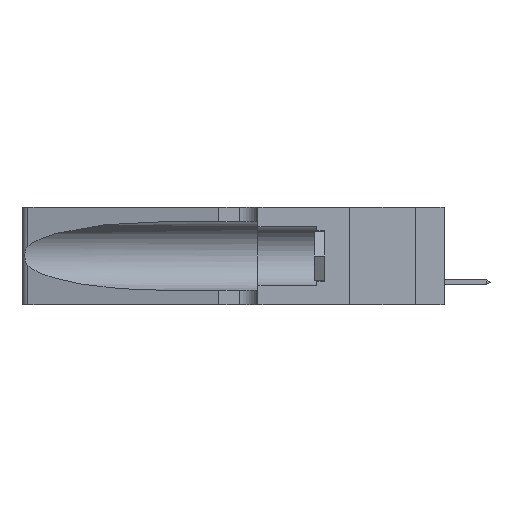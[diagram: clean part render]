
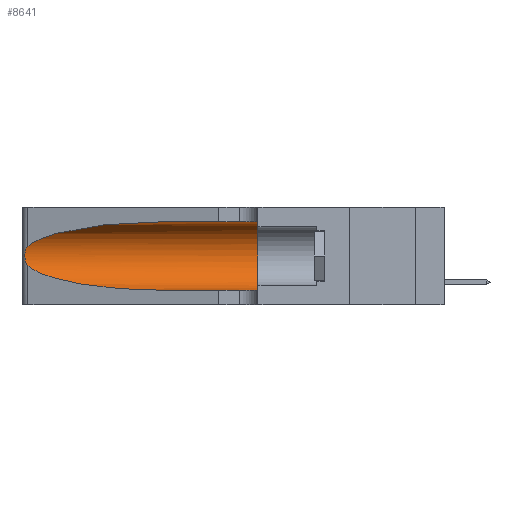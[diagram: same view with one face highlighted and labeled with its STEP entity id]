
A CAD part, left-side view. The second image highlights one B-rep face of the part: STEP entity #8641.
In plain terms, the highlighted cylindrical face has radius 3.308 mm (diameter 6.617 mm), a partial arc.
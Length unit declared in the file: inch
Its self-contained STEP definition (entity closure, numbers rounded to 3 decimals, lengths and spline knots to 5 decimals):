
#353 =( BOUNDED_CURVE ( )  B_SPLINE_CURVE ( 3, ( #4909, #16936, #8805, #553 ),
 .UNSPECIFIED., .F., .T. ) 
 B_SPLINE_CURVE_WITH_KNOTS ( ( 4, 4 ),
 ( 3.44316, 4.71239 ),
 .UNSPECIFIED. ) 
 CURVE ( )  GEOMETRIC_REPRESENTATION_ITEM ( )  RATIONAL_B_SPLINE_CURVE ( ( 1., 0.87, 0.87, 1. ) ) 
 REPRESENTATION_ITEM ( '' )  );
#553 = CARTESIAN_POINT ( 'NONE',  ( 0.1305, 0.72297, 0.05475 ) ) ;
#619 = ORIENTED_EDGE ( 'NONE', *, *, #15987, .F. ) ;
#901 = DIRECTION ( 'NONE',  ( 0., 0., -1. ) ) ;
#963 = CARTESIAN_POINT ( 'NONE',  ( 0.25789, 1.23486, 0.15765 ) ) ;
#1124 = CARTESIAN_POINT ( 'NONE',  ( 0.18966, 0.96281, 0.31525 ) ) ;
#1194 = ORIENTED_EDGE ( 'NONE', *, *, #21502, .F. ) ;
#1663 = VERTEX_POINT ( 'NONE', #10010 ) ;
#2228 = CARTESIAN_POINT ( 'NONE',  ( 0.1305, 0.35, 0.05475 ) ) ;
#2381 = DIRECTION ( 'NONE',  ( 0., -1., 0. ) ) ;
#2881 = CARTESIAN_POINT ( 'NONE',  ( 0.1305, 1.61858, 0.185 ) ) ;
#3036 = CARTESIAN_POINT ( 'NONE',  ( 0.25487, 1.22718, 0.22369 ) ) ;
#3123 = CARTESIAN_POINT ( 'NONE',  ( 0.26075, 1.23896, 0.19203 ) ) ;
#3367 = CARTESIAN_POINT ( 'NONE',  ( 0.25487, 1.22718, 0.22369 ) ) ;
#3397 = CARTESIAN_POINT ( 'NONE',  ( 0.26075, 1.23896, 0.178 ) ) ;
#3483 = LINE ( 'NONE', #20810, #13830 ) ;
#3526 = EDGE_LOOP ( 'NONE', ( #8559, #12706, #19933, #14990, #1194, #619 ) ) ;
#3646 = FACE_OUTER_BOUND ( 'NONE', #3526, .T. ) ;
#4675 =( BOUNDED_CURVE ( )  B_SPLINE_CURVE ( 3, ( #25642, #1124, #13586, #3367 ),
 .UNSPECIFIED., .F., .F. ) 
 B_SPLINE_CURVE_WITH_KNOTS ( ( 4, 4 ),
 ( 1.5708, 2.84003 ),
 .UNSPECIFIED. ) 
 CURVE ( )  GEOMETRIC_REPRESENTATION_ITEM ( )  RATIONAL_B_SPLINE_CURVE ( ( 1., 0.87, 0.87, 1. ) ) 
 REPRESENTATION_ITEM ( '' )  );
#4688 = AXIS2_PLACEMENT_3D ( 'NONE', #2881, #13170, #901 ) ;
#4909 = CARTESIAN_POINT ( 'NONE',  ( 0.25487, 1.22718, 0.14631 ) ) ;
#5129 = CARTESIAN_POINT ( 'NONE',  ( 0.25854, 1.2359, 0.20912 ) ) ;
#5323 = CARTESIAN_POINT ( 'NONE',  ( 0.25639, 1.23186, 0.15144 ) ) ;
#6638 = VERTEX_POINT ( 'NONE', #19495 ) ;
#7235 = DIRECTION ( 'NONE',  ( 0., 1., 0. ) ) ;
#7605 = CARTESIAN_POINT ( 'NONE',  ( 0.25555, 1.22994, 0.2215 ) ) ;
#8240 = CIRCLE ( 'NONE', #19545, 0.13025 ) ;
#8546 = DIRECTION ( 'NONE',  ( 0., -1., 0. ) ) ;
#8559 = ORIENTED_EDGE ( 'NONE', *, *, #23004, .T. ) ;
#8641 = ADVANCED_FACE ( 'NONE', ( #3646 ), #22967, .F. ) ;
#8805 = CARTESIAN_POINT ( 'NONE',  ( 0.18966, 0.96281, 0.05475 ) ) ;
#9613 = VERTEX_POINT ( 'NONE', #25275 ) ;
#9688 = LINE ( 'NONE', #22993, #12542 ) ;
#10010 = CARTESIAN_POINT ( 'NONE',  ( 0.1305, 0.35, 0.31525 ) ) ;
#11279 = CARTESIAN_POINT ( 'NONE',  ( 0.25487, 1.22718, 0.22369 ) ) ;
#11384 = DIRECTION ( 'NONE',  ( 0., 0., 1. ) ) ;
#11907 = CARTESIAN_POINT ( 'NONE',  ( 0.1305, 0.72297, 0.31525 ) ) ;
#12542 = VECTOR ( 'NONE', #2381, 39.37008 ) ;
#12706 = ORIENTED_EDGE ( 'NONE', *, *, #15152, .T. ) ;
#13170 = DIRECTION ( 'NONE',  ( 0., -1., 0. ) ) ;
#13586 = CARTESIAN_POINT ( 'NONE',  ( 0.2373, 1.15595, 0.28018 ) ) ;
#13830 = VECTOR ( 'NONE', #8546, 39.37008 ) ;
#14990 = ORIENTED_EDGE ( 'NONE', *, *, #25377, .T. ) ;
#15152 = EDGE_CURVE ( 'NONE', #15187, #6638, #19867, .T. ) ;
#15187 = VERTEX_POINT ( 'NONE', #3036 ) ;
#15987 = EDGE_CURVE ( 'NONE', #23667, #1663, #3483, .T. ) ;
#16936 = CARTESIAN_POINT ( 'NONE',  ( 0.2373, 1.15595, 0.08982 ) ) ;
#17822 = CARTESIAN_POINT ( 'NONE',  ( 0.25487, 1.22718, 0.14631 ) ) ;
#18416 = VERTEX_POINT ( 'NONE', #2228 ) ;
#19495 = CARTESIAN_POINT ( 'NONE',  ( 0.25487, 1.22718, 0.14631 ) ) ;
#19519 = CARTESIAN_POINT ( 'NONE',  ( 0.1305, 0.35, 0.185 ) ) ;
#19545 = AXIS2_PLACEMENT_3D ( 'NONE', #19519, #7235, #11384 ) ;
#19710 = CARTESIAN_POINT ( 'NONE',  ( 0.25856, 1.23593, 0.16098 ) ) ;
#19867 = B_SPLINE_CURVE_WITH_KNOTS ( 'NONE', 3,
 ( #11279, #7605, #21854, #25676, #5129, #25858, #3123, #3397, #19895, #19710, #963, #5323, #25580, #17822 ),
 .UNSPECIFIED., .F., .F.,
 ( 4, 2, 2, 2, 2, 2, 4 ),
 ( 0., 0.00027, 0.00053, 0.00107, 0.0016, 0.00187, 0.00214 ),
 .UNSPECIFIED. ) ;
#19895 = CARTESIAN_POINT ( 'NONE',  ( 0.26017, 1.23833, 0.17102 ) ) ;
#19933 = ORIENTED_EDGE ( 'NONE', *, *, #22103, .T. ) ;
#20810 = CARTESIAN_POINT ( 'NONE',  ( 0.1305, 1.61858, 0.31525 ) ) ;
#21502 = EDGE_CURVE ( 'NONE', #1663, #18416, #8240, .T. ) ;
#21854 = CARTESIAN_POINT ( 'NONE',  ( 0.25639, 1.23184, 0.21858 ) ) ;
#22103 = EDGE_CURVE ( 'NONE', #6638, #9613, #353, .T. ) ;
#22967 = CYLINDRICAL_SURFACE ( 'NONE', #4688, 0.13025 ) ;
#22993 = CARTESIAN_POINT ( 'NONE',  ( 0.1305, 1.61858, 0.05475 ) ) ;
#23004 = EDGE_CURVE ( 'NONE', #23667, #15187, #4675, .T. ) ;
#23667 = VERTEX_POINT ( 'NONE', #11907 ) ;
#25275 = CARTESIAN_POINT ( 'NONE',  ( 0.1305, 0.72297, 0.05475 ) ) ;
#25377 = EDGE_CURVE ( 'NONE', #9613, #18416, #9688, .T. ) ;
#25580 = CARTESIAN_POINT ( 'NONE',  ( 0.25555, 1.22993, 0.14849 ) ) ;
#25642 = CARTESIAN_POINT ( 'NONE',  ( 0.1305, 0.72297, 0.31525 ) ) ;
#25676 = CARTESIAN_POINT ( 'NONE',  ( 0.25787, 1.23484, 0.2124 ) ) ;
#25858 = CARTESIAN_POINT ( 'NONE',  ( 0.26018, 1.23835, 0.19895 ) ) ;
